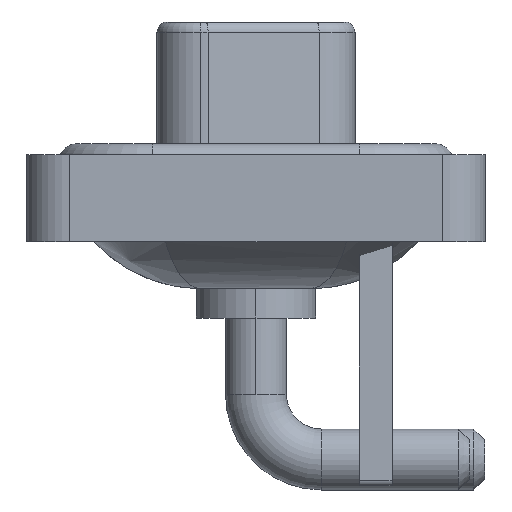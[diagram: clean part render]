
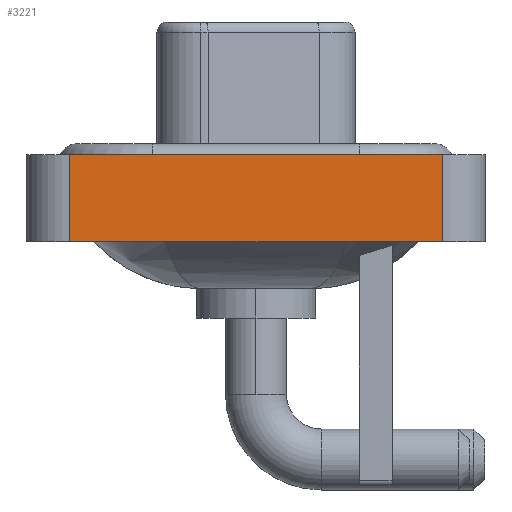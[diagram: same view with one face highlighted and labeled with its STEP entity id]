
A CAD part, left-side view. The second image highlights one B-rep face of the part: STEP entity #3221.
In plain terms, the highlighted planar face has unit normal (-1, 0, 0).
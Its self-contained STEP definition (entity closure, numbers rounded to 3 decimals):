
#780 = LINE ( 'NONE', #17803, #12290 ) ;
#1264 = EDGE_CURVE ( 'NONE', #3198, #14984, #780, .T. ) ;
#1342 = VECTOR ( 'NONE', #3909, 1000. ) ;
#2678 = FACE_OUTER_BOUND ( 'NONE', #8768, .T. ) ;
#2825 = DIRECTION ( 'NONE',  ( 0., 0., 1. ) ) ;
#3198 = VERTEX_POINT ( 'NONE', #7412 ) ;
#3221 = ADVANCED_FACE ( 'NONE', ( #2678 ), #8848, .T. ) ;
#3307 = ORIENTED_EDGE ( 'NONE', *, *, #5456, .F. ) ;
#3808 = CARTESIAN_POINT ( 'NONE',  ( -7.3, -8.55, -3.6 ) ) ;
#3909 = DIRECTION ( 'NONE',  ( 0., 0., 1. ) ) ;
#4036 = DIRECTION ( 'NONE',  ( 0., -1., 0. ) ) ;
#4116 = EDGE_CURVE ( 'NONE', #19091, #14217, #7370, .T. ) ;
#4242 = CARTESIAN_POINT ( 'NONE',  ( -7.3, 8.55, -3.6 ) ) ;
#4287 = DIRECTION ( 'NONE',  ( 0., 0., 1. ) ) ;
#4733 = ORIENTED_EDGE ( 'NONE', *, *, #4116, .F. ) ;
#5456 = EDGE_CURVE ( 'NONE', #3198, #19091, #16411, .T. ) ;
#5777 = CARTESIAN_POINT ( 'NONE',  ( -7.3, -8.55, 0.4 ) ) ;
#6910 = CARTESIAN_POINT ( 'NONE',  ( -7.3, -8.55, -3.6 ) ) ;
#6976 = ORIENTED_EDGE ( 'NONE', *, *, #1264, .T. ) ;
#7054 = DIRECTION ( 'NONE',  ( 0., -1., 0. ) ) ;
#7274 = CARTESIAN_POINT ( 'NONE',  ( -7.3, -8.55, 0.4 ) ) ;
#7370 = LINE ( 'NONE', #7274, #18914 ) ;
#7412 = CARTESIAN_POINT ( 'NONE',  ( -7.3, 8.55, -3.6 ) ) ;
#8508 = ORIENTED_EDGE ( 'NONE', *, *, #18303, .T. ) ;
#8768 = EDGE_LOOP ( 'NONE', ( #8508, #4733, #3307, #6976 ) ) ;
#8848 = PLANE ( 'NONE',  #20001 ) ;
#11522 = LINE ( 'NONE', #3808, #1342 ) ;
#11981 = CARTESIAN_POINT ( 'NONE',  ( -7.3, -8.55, -3.6 ) ) ;
#12290 = VECTOR ( 'NONE', #7054, 1000. ) ;
#14217 = VERTEX_POINT ( 'NONE', #5777 ) ;
#14984 = VERTEX_POINT ( 'NONE', #6910 ) ;
#16411 = LINE ( 'NONE', #4242, #16704 ) ;
#16704 = VECTOR ( 'NONE', #2825, 1000. ) ;
#17211 = CARTESIAN_POINT ( 'NONE',  ( -7.3, 8.55, 0.4 ) ) ;
#17803 = CARTESIAN_POINT ( 'NONE',  ( -7.3, -8.55, -3.6 ) ) ;
#18178 = DIRECTION ( 'NONE',  ( -1., 0., 0. ) ) ;
#18303 = EDGE_CURVE ( 'NONE', #14984, #14217, #11522, .T. ) ;
#18914 = VECTOR ( 'NONE', #4036, 1000. ) ;
#19091 = VERTEX_POINT ( 'NONE', #17211 ) ;
#20001 = AXIS2_PLACEMENT_3D ( 'NONE', #11981, #18178, #4287 ) ;
